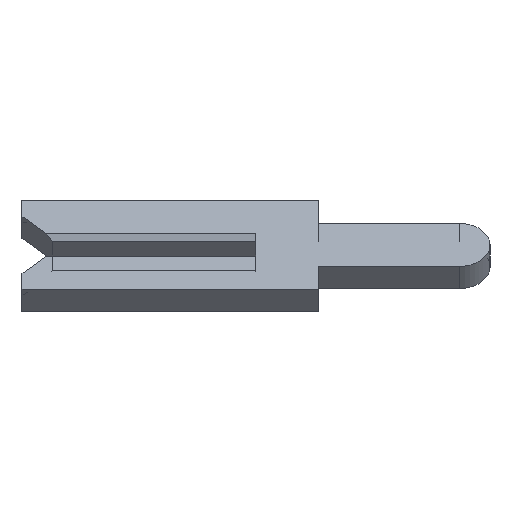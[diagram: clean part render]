
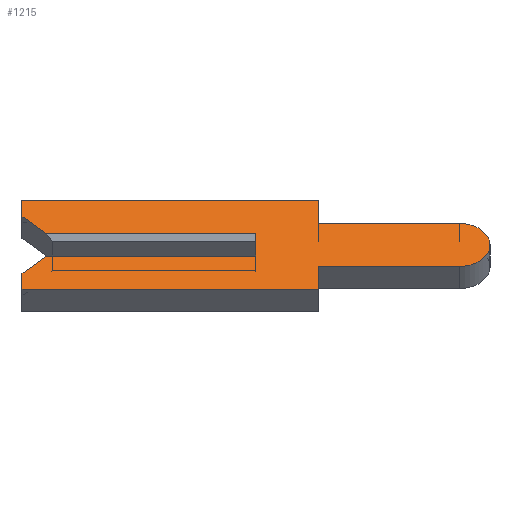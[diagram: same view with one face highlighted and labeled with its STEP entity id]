
A CAD part, left-side view. The second image highlights one B-rep face of the part: STEP entity #1215.
In plain terms, the highlighted face is planar.
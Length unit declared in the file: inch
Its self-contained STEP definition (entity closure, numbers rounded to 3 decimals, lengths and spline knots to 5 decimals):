
#4 = DIRECTION ( 'NONE',  ( 0., 0., -1. ) ) ;
#14 = EDGE_CURVE ( 'NONE', #438, #1596, #392, .T. ) ;
#42 = EDGE_CURVE ( 'NONE', #264, #143, #102, .T. ) ;
#44 = CARTESIAN_POINT ( 'NONE',  ( -0.01, 0.15, 0.026 ) ) ;
#52 = CARTESIAN_POINT ( 'NONE',  ( -0.01, 0.15, -0.04 ) ) ;
#72 = DIRECTION ( 'NONE',  ( 0., 1., 0. ) ) ;
#74 = ORIENTED_EDGE ( 'NONE', *, *, #1336, .F. ) ;
#94 = CARTESIAN_POINT ( 'NONE',  ( -0.01, -0.04, -0.0195 ) ) ;
#99 = VERTEX_POINT ( 'NONE', #1756 ) ;
#102 = LINE ( 'NONE', #1042, #1009 ) ;
#143 = VERTEX_POINT ( 'NONE', #52 ) ;
#191 = CARTESIAN_POINT ( 'NONE',  ( -0.01, 0.15, 0.01 ) ) ;
#195 = LINE ( 'NONE', #518, #1316 ) ;
#206 = CARTESIAN_POINT ( 'NONE',  ( -0.01, 0.1305, -0.0065 ) ) ;
#212 = CARTESIAN_POINT ( 'NONE',  ( -0.01, 0.15, -0.026 ) ) ;
#214 = ORIENTED_EDGE ( 'NONE', *, *, #1124, .F. ) ;
#223 = EDGE_CURVE ( 'NONE', #241, #1092, #1161, .T. ) ;
#230 = DIRECTION ( 'NONE',  ( 0., 0., -1. ) ) ;
#241 = VERTEX_POINT ( 'NONE', #1593 ) ;
#264 = VERTEX_POINT ( 'NONE', #626 ) ;
#273 = EDGE_CURVE ( 'NONE', #1385, #1116, #414, .T. ) ;
#304 = VECTOR ( 'NONE', #1348, 39.37008 ) ;
#326 = CARTESIAN_POINT ( 'NONE',  ( -0.01, -0.04, -0.0195 ) ) ;
#339 = CARTESIAN_POINT ( 'NONE',  ( -0.01, 0.1305, 0.0065 ) ) ;
#345 = DIRECTION ( 'NONE',  ( 0., 0., 1. ) ) ;
#348 = CARTESIAN_POINT ( 'NONE',  ( -0.01, 0.15, 0.04 ) ) ;
#389 = VERTEX_POINT ( 'NONE', #931 ) ;
#392 = LINE ( 'NONE', #326, #1470 ) ;
#396 = EDGE_CURVE ( 'NONE', #1596, #264, #1716, .T. ) ;
#414 = LINE ( 'NONE', #206, #304 ) ;
#431 = LINE ( 'NONE', #339, #1105 ) ;
#438 = VERTEX_POINT ( 'NONE', #1285 ) ;
#469 = DIRECTION ( 'NONE',  ( 0., 0., 1. ) ) ;
#488 = EDGE_CURVE ( 'NONE', #1116, #802, #732, .T. ) ;
#495 = ORIENTED_EDGE ( 'NONE', *, *, #1502, .F. ) ;
#501 = ORIENTED_EDGE ( 'NONE', *, *, #273, .F. ) ;
#507 = DIRECTION ( 'NONE',  ( 0., -1., 0. ) ) ;
#508 = VECTOR ( 'NONE', #230, 39.37008 ) ;
#513 = CARTESIAN_POINT ( 'NONE',  ( -0.01, -0.04, 0.04 ) ) ;
#518 = CARTESIAN_POINT ( 'NONE',  ( -0.01, 0.15, 0.04 ) ) ;
#525 = DIRECTION ( 'NONE',  ( 0., 0., -1. ) ) ;
#559 = CARTESIAN_POINT ( 'NONE',  ( -0.01, -0.1305, -0.01 ) ) ;
#565 = LINE ( 'NONE', #1033, #865 ) ;
#586 = CARTESIAN_POINT ( 'NONE',  ( -0.01, 0., 0.01 ) ) ;
#610 = AXIS2_PLACEMENT_3D ( 'NONE', #1612, #1184, #637 ) ;
#626 = CARTESIAN_POINT ( 'NONE',  ( -0.01, -0.04, -0.04 ) ) ;
#629 = PLANE ( 'NONE',  #610 ) ;
#637 = DIRECTION ( 'NONE',  ( 0., 0., -1. ) ) ;
#732 = LINE ( 'NONE', #559, #858 ) ;
#742 = ORIENTED_EDGE ( 'NONE', *, *, #396, .F. ) ;
#751 = CARTESIAN_POINT ( 'NONE',  ( -0.01, 0., 0.0065 ) ) ;
#771 = DIRECTION ( 'NONE',  ( 0., 0.707, 0.707 ) ) ;
#789 = DIRECTION ( 'NONE',  ( 1., 0., 0. ) ) ;
#802 = VERTEX_POINT ( 'NONE', #872 ) ;
#846 = DIRECTION ( 'NONE',  ( 0., -1., 0. ) ) ;
#858 = VECTOR ( 'NONE', #846, 39.37008 ) ;
#865 = VECTOR ( 'NONE', #1749, 39.37008 ) ;
#872 = CARTESIAN_POINT ( 'NONE',  ( -0.01, 0., -0.01 ) ) ;
#878 = LINE ( 'NONE', #935, #508 ) ;
#888 = LINE ( 'NONE', #212, #1420 ) ;
#931 = CARTESIAN_POINT ( 'NONE',  ( -0.01, -0.04, 0.0195 ) ) ;
#935 = CARTESIAN_POINT ( 'NONE',  ( -0.01, -0.04, 0.04 ) ) ;
#938 = CIRCLE ( 'NONE', #1454, 0.0195 ) ;
#960 = EDGE_CURVE ( 'NONE', #802, #1112, #1547, .T. ) ;
#973 = VECTOR ( 'NONE', #469, 39.37008 ) ;
#1009 = VECTOR ( 'NONE', #1323, 39.37008 ) ;
#1023 = ORIENTED_EDGE ( 'NONE', *, *, #1373, .T. ) ;
#1033 = CARTESIAN_POINT ( 'NONE',  ( -0.01, -0.04, 0.0195 ) ) ;
#1042 = CARTESIAN_POINT ( 'NONE',  ( -0.01, 0.15, -0.04 ) ) ;
#1045 = CARTESIAN_POINT ( 'NONE',  ( -0.01, 0.15, -0.026 ) ) ;
#1063 = DIRECTION ( 'NONE',  ( 0., 0., 1. ) ) ;
#1092 = VERTEX_POINT ( 'NONE', #348 ) ;
#1105 = VECTOR ( 'NONE', #771, 39.37008 ) ;
#1109 = CARTESIAN_POINT ( 'NONE',  ( -0.01, -0.04, -0.04 ) ) ;
#1112 = VERTEX_POINT ( 'NONE', #586 ) ;
#1113 = VECTOR ( 'NONE', #345, 39.37008 ) ;
#1116 = VERTEX_POINT ( 'NONE', #1739 ) ;
#1124 = EDGE_CURVE ( 'NONE', #389, #1706, #565, .T. ) ;
#1136 = ORIENTED_EDGE ( 'NONE', *, *, #1310, .F. ) ;
#1161 = LINE ( 'NONE', #44, #1113 ) ;
#1182 = ORIENTED_EDGE ( 'NONE', *, *, #14, .F. ) ;
#1184 = DIRECTION ( 'NONE',  ( 1., 0., 0. ) ) ;
#1215 = ADVANCED_FACE ( 'NONE', ( #1244 ), #629, .F. ) ;
#1238 = VECTOR ( 'NONE', #4, 39.37008 ) ;
#1244 = FACE_OUTER_BOUND ( 'NONE', #1578, .T. ) ;
#1285 = CARTESIAN_POINT ( 'NONE',  ( -0.01, -0.1305, -0.0195 ) ) ;
#1310 = EDGE_CURVE ( 'NONE', #99, #241, #431, .T. ) ;
#1316 = VECTOR ( 'NONE', #507, 39.37008 ) ;
#1323 = DIRECTION ( 'NONE',  ( 0., 1., 0. ) ) ;
#1336 = EDGE_CURVE ( 'NONE', #143, #1385, #888, .T. ) ;
#1348 = DIRECTION ( 'NONE',  ( 0., -0.707, 0.707 ) ) ;
#1373 = EDGE_CURVE ( 'NONE', #99, #1112, #1742, .T. ) ;
#1376 = VECTOR ( 'NONE', #1461, 39.37008 ) ;
#1385 = VERTEX_POINT ( 'NONE', #1045 ) ;
#1403 = ORIENTED_EDGE ( 'NONE', *, *, #42, .F. ) ;
#1420 = VECTOR ( 'NONE', #1063, 39.37008 ) ;
#1448 = VERTEX_POINT ( 'NONE', #513 ) ;
#1454 = AXIS2_PLACEMENT_3D ( 'NONE', #1629, #789, #525 ) ;
#1461 = DIRECTION ( 'NONE',  ( 0., -1., 0. ) ) ;
#1463 = ORIENTED_EDGE ( 'NONE', *, *, #223, .F. ) ;
#1470 = VECTOR ( 'NONE', #72, 39.37008 ) ;
#1502 = EDGE_CURVE ( 'NONE', #1092, #1448, #195, .T. ) ;
#1525 = EDGE_CURVE ( 'NONE', #1448, #389, #878, .T. ) ;
#1532 = ORIENTED_EDGE ( 'NONE', *, *, #960, .F. ) ;
#1547 = LINE ( 'NONE', #751, #973 ) ;
#1578 = EDGE_LOOP ( 'NONE', ( #1023, #1532, #1726, #501, #74, #1403, #742, #1182, #1727, #214, #1773, #495, #1463, #1136 ) ) ;
#1590 = EDGE_CURVE ( 'NONE', #1706, #438, #938, .T. ) ;
#1593 = CARTESIAN_POINT ( 'NONE',  ( -0.01, 0.15, 0.026 ) ) ;
#1596 = VERTEX_POINT ( 'NONE', #94 ) ;
#1612 = CARTESIAN_POINT ( 'NONE',  ( -0.01, -0.1305, 0. ) ) ;
#1629 = CARTESIAN_POINT ( 'NONE',  ( -0.01, -0.1305, 0. ) ) ;
#1706 = VERTEX_POINT ( 'NONE', #1767 ) ;
#1716 = LINE ( 'NONE', #1109, #1238 ) ;
#1726 = ORIENTED_EDGE ( 'NONE', *, *, #488, .F. ) ;
#1727 = ORIENTED_EDGE ( 'NONE', *, *, #1590, .F. ) ;
#1739 = CARTESIAN_POINT ( 'NONE',  ( -0.01, 0.134, -0.01 ) ) ;
#1742 = LINE ( 'NONE', #191, #1376 ) ;
#1749 = DIRECTION ( 'NONE',  ( 0., -1., 0. ) ) ;
#1756 = CARTESIAN_POINT ( 'NONE',  ( -0.01, 0.134, 0.01 ) ) ;
#1767 = CARTESIAN_POINT ( 'NONE',  ( -0.01, -0.1305, 0.0195 ) ) ;
#1773 = ORIENTED_EDGE ( 'NONE', *, *, #1525, .F. ) ;
